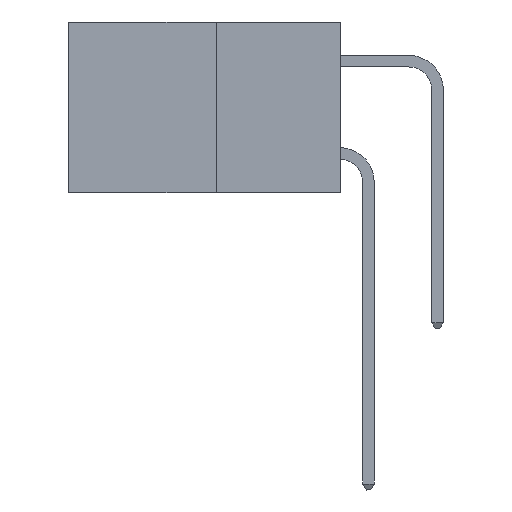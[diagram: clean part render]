
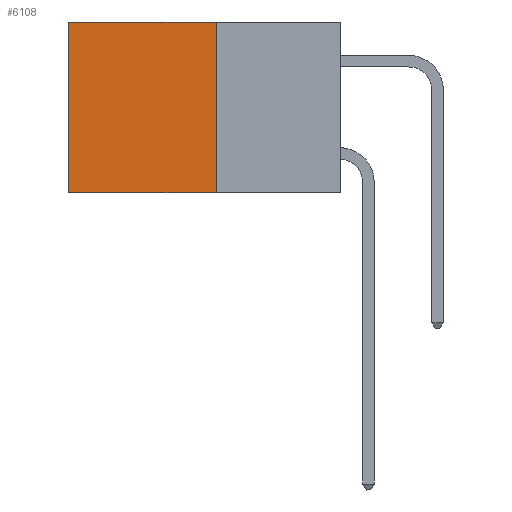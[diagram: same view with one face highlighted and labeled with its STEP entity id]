
A CAD part, left-side view. The second image highlights one B-rep face of the part: STEP entity #6108.
In plain terms, the highlighted planar face has unit normal (-1, 0, 0).
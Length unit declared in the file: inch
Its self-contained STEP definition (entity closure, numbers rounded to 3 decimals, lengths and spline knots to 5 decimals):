
#122 = VECTOR ( 'NONE', #8343, 39.37008 ) ;
#741 = DIRECTION ( 'NONE',  ( 0., 1., 0. ) ) ;
#1407 = DIRECTION ( 'NONE',  ( 1., 0., 0. ) ) ;
#1419 = DIRECTION ( 'NONE',  ( 0., 0., -1. ) ) ;
#1595 = CARTESIAN_POINT ( 'NONE',  ( 0.277, 0.27, -0.37 ) ) ;
#1628 = DIRECTION ( 'NONE',  ( 0., 1., 0. ) ) ;
#1651 = PLANE ( 'NONE',  #2750 ) ;
#1662 = CARTESIAN_POINT ( 'NONE',  ( 0.277, 0.27, -0.37 ) ) ;
#1707 = VERTEX_POINT ( 'NONE', #4461 ) ;
#1723 = EDGE_CURVE ( 'NONE', #10798, #1707, #6806, .T. ) ;
#1922 = ORIENTED_EDGE ( 'NONE', *, *, #1723, .F. ) ;
#2063 = EDGE_CURVE ( 'NONE', #2354, #10798, #3706, .T. ) ;
#2127 = CARTESIAN_POINT ( 'NONE',  ( 0.277, 0.27, 0. ) ) ;
#2354 = VERTEX_POINT ( 'NONE', #2127 ) ;
#2389 = ORIENTED_EDGE ( 'NONE', *, *, #2063, .F. ) ;
#2750 = AXIS2_PLACEMENT_3D ( 'NONE', #1662, #1407, #1419 ) ;
#2844 = ORIENTED_EDGE ( 'NONE', *, *, #6102, .T. ) ;
#3064 = CARTESIAN_POINT ( 'NONE',  ( 0.277, 0.27, -0.37 ) ) ;
#3288 = VECTOR ( 'NONE', #1628, 39.37008 ) ;
#3706 = LINE ( 'NONE', #1595, #122 ) ;
#4461 = CARTESIAN_POINT ( 'NONE',  ( 0.277, 0.59, -0.37 ) ) ;
#5910 = FACE_OUTER_BOUND ( 'NONE', #8236, .T. ) ;
#5973 = EDGE_CURVE ( 'NONE', #7947, #1707, #10156, .T. ) ;
#6082 = ORIENTED_EDGE ( 'NONE', *, *, #5973, .T. ) ;
#6102 = EDGE_CURVE ( 'NONE', #2354, #7947, #11205, .T. ) ;
#6104 = CARTESIAN_POINT ( 'NONE',  ( 0.277, 0.27, 0. ) ) ;
#6108 = ADVANCED_FACE ( 'NONE', ( #5910 ), #1651, .F. ) ;
#6332 = CARTESIAN_POINT ( 'NONE',  ( 0.277, 0.27, -0.37 ) ) ;
#6806 = LINE ( 'NONE', #6332, #8867 ) ;
#7480 = VECTOR ( 'NONE', #7754, 39.37008 ) ;
#7724 = CARTESIAN_POINT ( 'NONE',  ( 0.277, 0.59, -0.37 ) ) ;
#7754 = DIRECTION ( 'NONE',  ( 0., 0., -1. ) ) ;
#7947 = VERTEX_POINT ( 'NONE', #9792 ) ;
#8236 = EDGE_LOOP ( 'NONE', ( #6082, #1922, #2389, #2844 ) ) ;
#8343 = DIRECTION ( 'NONE',  ( 0., 0., -1. ) ) ;
#8867 = VECTOR ( 'NONE', #741, 39.37008 ) ;
#9792 = CARTESIAN_POINT ( 'NONE',  ( 0.277, 0.59, 0. ) ) ;
#10156 = LINE ( 'NONE', #7724, #7480 ) ;
#10798 = VERTEX_POINT ( 'NONE', #3064 ) ;
#11205 = LINE ( 'NONE', #6104, #3288 ) ;
